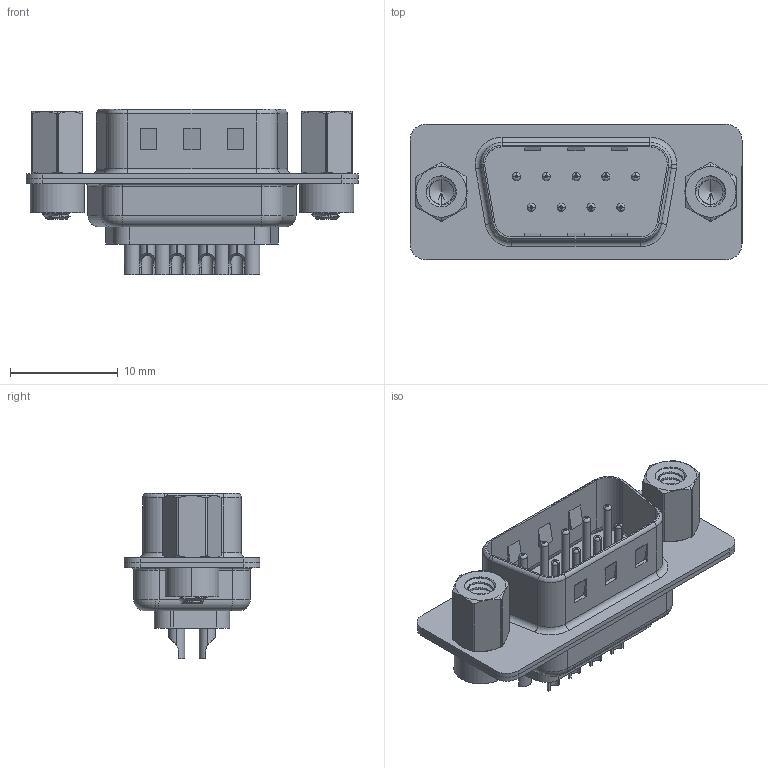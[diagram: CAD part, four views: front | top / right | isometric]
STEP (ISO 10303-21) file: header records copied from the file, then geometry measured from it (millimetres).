
FILE_DESCRIPTION (( 'STEP AP203' ), '1' );
FILE_NAME ('627-009-222-543.STEP', '2018-10-03T15:17:44', ( '' ), ( '' ), 'SwSTEP 2.0', 'SolidWorks 2016', '' );
FILE_SCHEMA (( 'CONFIG_CONTROL_DESIGN' ));
Length unit declared in the file: millimetre
Products named in the file (8): 627-009-222-543; 627 Housing_09 LP; 627 Shell Front_09 Contacts; 627 Shell Rear_09 Contacts; 627 Contact Row 1_22L; 627 Contact Row 2_22L; 627 4-40 Threaded Rivet; 627 4-40 Hex Standoff
Assembly tree (16 placements, depth 2):
  627-009-222-543
    627 Housing_09 LP
    627 Shell Front_09 Contacts
    627 Shell Rear_09 Contacts
    627 Contact Row 1_22L  x5
    627 Contact Row 2_22L  x4
    627 4-40 Threaded Rivet  x2
    627 4-40 Hex Standoff  x2
Bounding box: 30.8 x 12.6 x 15.35 mm (x, y, z)
Volume: 1529.7 mm3; surface area: 4441.9 mm2
Topology: 16 solids, 16 shells, 1006 faces, 2583 edges, 1638 vertices
Faces by surface type: cylinder 462, plane 255, torus 245, cone 26, bspline 18
Entity records: 20914 total; most frequent: CARTESIAN_POINT 7206, DIRECTION 2776, ORIENTED_EDGE 2606, EDGE_CURVE 1303, AXIS2_PLACEMENT_3D 1109, VERTEX_POINT 828, EDGE_LOOP 591, CIRCLE 581
